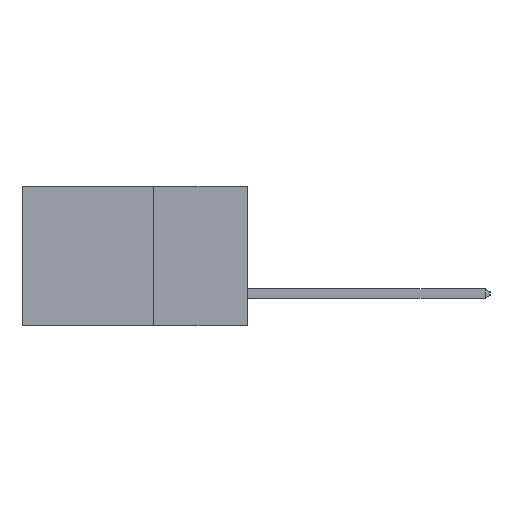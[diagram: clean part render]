
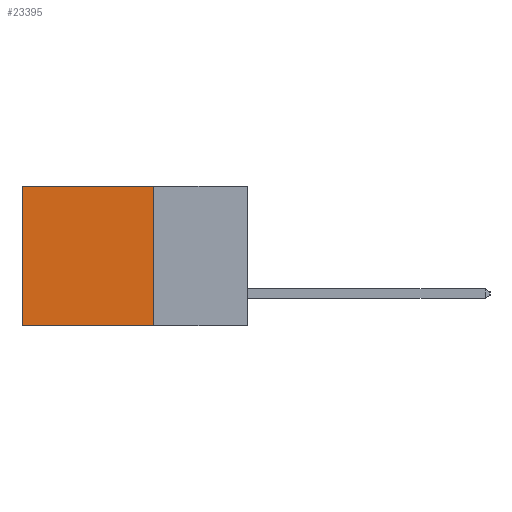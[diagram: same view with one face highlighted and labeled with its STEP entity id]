
A CAD part, left-side view. The second image highlights one B-rep face of the part: STEP entity #23395.
In plain terms, the highlighted planar face has unit normal (-1, 0, 0).
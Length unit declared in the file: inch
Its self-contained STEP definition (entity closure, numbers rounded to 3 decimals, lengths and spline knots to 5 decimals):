
#110 = VERTEX_POINT ( 'NONE', #6252 ) ;
#817 = FACE_OUTER_BOUND ( 'NONE', #11264, .T. ) ;
#2761 = ORIENTED_EDGE ( 'NONE', *, *, #8931, .T. ) ;
#2953 = PLANE ( 'NONE',  #14737 ) ;
#3213 = VECTOR ( 'NONE', #12801, 39.37008 ) ;
#4439 = DIRECTION ( 'NONE',  ( 0., 1., 0. ) ) ;
#5744 = CARTESIAN_POINT ( 'NONE',  ( 0.2615, 0.6, 0. ) ) ;
#6039 = LINE ( 'NONE', #12160, #10964 ) ;
#6252 = CARTESIAN_POINT ( 'NONE',  ( 0.2615, 0.6, -0.37 ) ) ;
#6920 = VERTEX_POINT ( 'NONE', #10618 ) ;
#8155 = LINE ( 'NONE', #18240, #3213 ) ;
#8597 = LINE ( 'NONE', #13656, #22038 ) ;
#8845 = DIRECTION ( 'NONE',  ( 0., 0., -1. ) ) ;
#8931 = EDGE_CURVE ( 'NONE', #22424, #13602, #8155, .T. ) ;
#10618 = CARTESIAN_POINT ( 'NONE',  ( 0.2615, 0.25, -0.37 ) ) ;
#10964 = VECTOR ( 'NONE', #21226, 39.37008 ) ;
#11169 = ORIENTED_EDGE ( 'NONE', *, *, #18662, .F. ) ;
#11220 = LINE ( 'NONE', #13989, #14991 ) ;
#11264 = EDGE_LOOP ( 'NONE', ( #13069, #14414, #11169, #2761 ) ) ;
#11280 = CARTESIAN_POINT ( 'NONE',  ( 0.2615, 0.25, 0. ) ) ;
#12160 = CARTESIAN_POINT ( 'NONE',  ( 0.2615, 0.25, -0.37 ) ) ;
#12801 = DIRECTION ( 'NONE',  ( 0., 1., 0. ) ) ;
#13069 = ORIENTED_EDGE ( 'NONE', *, *, #19291, .T. ) ;
#13602 = VERTEX_POINT ( 'NONE', #5744 ) ;
#13656 = CARTESIAN_POINT ( 'NONE',  ( 0.2615, 0.25, -0.37 ) ) ;
#13989 = CARTESIAN_POINT ( 'NONE',  ( 0.2615, 0.6, -0.37 ) ) ;
#14083 = CARTESIAN_POINT ( 'NONE',  ( 0.2615, 0.25, -0.37 ) ) ;
#14414 = ORIENTED_EDGE ( 'NONE', *, *, #19171, .F. ) ;
#14737 = AXIS2_PLACEMENT_3D ( 'NONE', #14083, #19839, #8845 ) ;
#14991 = VECTOR ( 'NONE', #15830, 39.37008 ) ;
#15830 = DIRECTION ( 'NONE',  ( 0., 0., -1. ) ) ;
#18240 = CARTESIAN_POINT ( 'NONE',  ( 0.2615, 0.25, 0. ) ) ;
#18662 = EDGE_CURVE ( 'NONE', #22424, #6920, #6039, .T. ) ;
#19171 = EDGE_CURVE ( 'NONE', #6920, #110, #8597, .T. ) ;
#19291 = EDGE_CURVE ( 'NONE', #13602, #110, #11220, .T. ) ;
#19839 = DIRECTION ( 'NONE',  ( 1., 0., 0. ) ) ;
#21226 = DIRECTION ( 'NONE',  ( 0., 0., -1. ) ) ;
#22038 = VECTOR ( 'NONE', #4439, 39.37008 ) ;
#22424 = VERTEX_POINT ( 'NONE', #11280 ) ;
#23395 = ADVANCED_FACE ( 'NONE', ( #817 ), #2953, .F. ) ;
